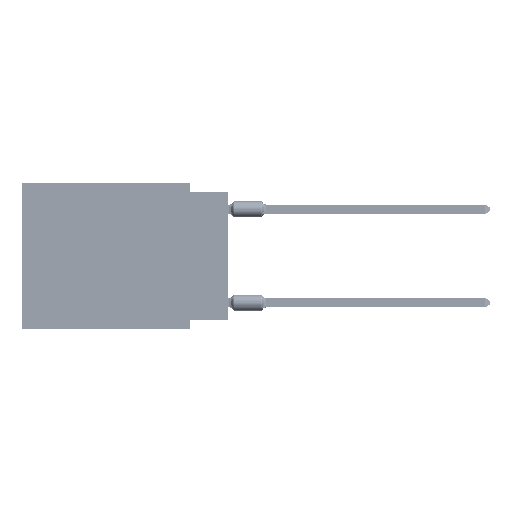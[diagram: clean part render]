
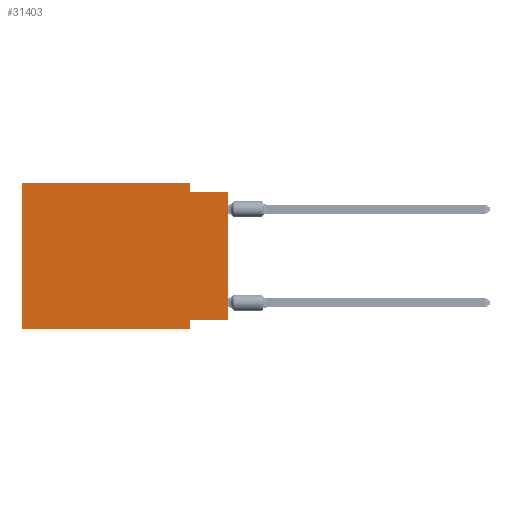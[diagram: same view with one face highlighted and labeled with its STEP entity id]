
A CAD part, left-side view. The second image highlights one B-rep face of the part: STEP entity #31403.
In plain terms, the highlighted planar face has unit normal (-1, 0, 0).
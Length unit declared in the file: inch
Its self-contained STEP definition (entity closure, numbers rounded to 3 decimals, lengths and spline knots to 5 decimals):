
#502 = CARTESIAN_POINT ( 'NONE',  ( 0., 0.1, 0. ) ) ;
#776 = CARTESIAN_POINT ( 'NONE',  ( 0., 0.1, -0.365 ) ) ;
#871 = ORIENTED_EDGE ( 'NONE', *, *, #56005, .F. ) ;
#4397 = DIRECTION ( 'NONE',  ( 0., 0., 1. ) ) ;
#8468 = EDGE_CURVE ( 'NONE', #18296, #77233, #19680, .T. ) ;
#9957 = VERTEX_POINT ( 'NONE', #20885 ) ;
#13483 = DIRECTION ( 'NONE',  ( 0., 0., -1. ) ) ;
#15169 = PLANE ( 'NONE',  #75862 ) ;
#15532 = LINE ( 'NONE', #53945, #24849 ) ;
#15560 = LINE ( 'NONE', #70926, #29838 ) ;
#15585 = DIRECTION ( 'NONE',  ( 0., 0., -1. ) ) ;
#15783 = EDGE_CURVE ( 'NONE', #9957, #73552, #64071, .T. ) ;
#18296 = VERTEX_POINT ( 'NONE', #776 ) ;
#18966 = VERTEX_POINT ( 'NONE', #61311 ) ;
#19308 = CARTESIAN_POINT ( 'NONE',  ( 0., 0.1, -0.39 ) ) ;
#19680 = LINE ( 'NONE', #44871, #29860 ) ;
#19714 = VERTEX_POINT ( 'NONE', #60621 ) ;
#20586 = ORIENTED_EDGE ( 'NONE', *, *, #8468, .F. ) ;
#20684 = CARTESIAN_POINT ( 'NONE',  ( 0., 0.55, 0. ) ) ;
#20786 = DIRECTION ( 'NONE',  ( 0., -1., 0. ) ) ;
#20885 = CARTESIAN_POINT ( 'NONE',  ( 0., 0.55, 0. ) ) ;
#21178 = ORIENTED_EDGE ( 'NONE', *, *, #34280, .T. ) ;
#21198 = CARTESIAN_POINT ( 'NONE',  ( 0., 0.55, -0.39 ) ) ;
#22147 = DIRECTION ( 'NONE',  ( 0., -1., 0. ) ) ;
#22645 = VERTEX_POINT ( 'NONE', #48712 ) ;
#23560 = VECTOR ( 'NONE', #75396, 39.37008 ) ;
#24849 = VECTOR ( 'NONE', #34932, 39.37008 ) ;
#27950 = CARTESIAN_POINT ( 'NONE',  ( 0., 0.55, 0. ) ) ;
#29838 = VECTOR ( 'NONE', #22147, 39.37008 ) ;
#29860 = VECTOR ( 'NONE', #13483, 39.37008 ) ;
#30438 = LINE ( 'NONE', #55647, #67499 ) ;
#30782 = CARTESIAN_POINT ( 'NONE',  ( 0., 0.1, 0. ) ) ;
#31403 = ADVANCED_FACE ( 'NONE', ( #59766 ), #15169, .F. ) ;
#33748 = DIRECTION ( 'NONE',  ( 1., 0., 0. ) ) ;
#34280 = EDGE_CURVE ( 'NONE', #19714, #48058, #78796, .T. ) ;
#34932 = DIRECTION ( 'NONE',  ( 0., 0., 1. ) ) ;
#34978 = CARTESIAN_POINT ( 'NONE',  ( 0., 0., 0. ) ) ;
#36949 = EDGE_CURVE ( 'NONE', #73552, #22645, #68393, .T. ) ;
#37824 = VECTOR ( 'NONE', #4397, 39.37008 ) ;
#40198 = LINE ( 'NONE', #21198, #44003 ) ;
#42339 = ORIENTED_EDGE ( 'NONE', *, *, #52269, .T. ) ;
#44003 = VECTOR ( 'NONE', #20786, 39.37008 ) ;
#44871 = CARTESIAN_POINT ( 'NONE',  ( 0., 0.1, -0.39 ) ) ;
#48058 = VERTEX_POINT ( 'NONE', #59655 ) ;
#48712 = CARTESIAN_POINT ( 'NONE',  ( 0., 0.1, -0.025 ) ) ;
#48901 = VECTOR ( 'NONE', #71110, 39.37008 ) ;
#51818 = EDGE_LOOP ( 'NONE', ( #21178, #871, #59038, #57546, #54740, #42339, #20586, #59491 ) ) ;
#52269 = EDGE_CURVE ( 'NONE', #18966, #77233, #40198, .T. ) ;
#53945 = CARTESIAN_POINT ( 'NONE',  ( 0., 0.55, 0. ) ) ;
#54740 = ORIENTED_EDGE ( 'NONE', *, *, #58139, .F. ) ;
#55647 = CARTESIAN_POINT ( 'NONE',  ( 0., 0., -0.365 ) ) ;
#56005 = EDGE_CURVE ( 'NONE', #22645, #48058, #15560, .T. ) ;
#57546 = ORIENTED_EDGE ( 'NONE', *, *, #15783, .F. ) ;
#58139 = EDGE_CURVE ( 'NONE', #18966, #9957, #15532, .T. ) ;
#59038 = ORIENTED_EDGE ( 'NONE', *, *, #36949, .F. ) ;
#59491 = ORIENTED_EDGE ( 'NONE', *, *, #73820, .F. ) ;
#59655 = CARTESIAN_POINT ( 'NONE',  ( 0., 0., -0.025 ) ) ;
#59766 = FACE_OUTER_BOUND ( 'NONE', #51818, .T. ) ;
#60621 = CARTESIAN_POINT ( 'NONE',  ( 0., 0., -0.365 ) ) ;
#61311 = CARTESIAN_POINT ( 'NONE',  ( 0., 0.55, -0.39 ) ) ;
#64071 = LINE ( 'NONE', #20684, #48901 ) ;
#67499 = VECTOR ( 'NONE', #71488, 39.37008 ) ;
#68393 = LINE ( 'NONE', #30782, #23560 ) ;
#70926 = CARTESIAN_POINT ( 'NONE',  ( 0., 0., -0.025 ) ) ;
#71110 = DIRECTION ( 'NONE',  ( 0., -1., 0. ) ) ;
#71488 = DIRECTION ( 'NONE',  ( 0., 1., 0. ) ) ;
#73552 = VERTEX_POINT ( 'NONE', #502 ) ;
#73820 = EDGE_CURVE ( 'NONE', #19714, #18296, #30438, .T. ) ;
#75396 = DIRECTION ( 'NONE',  ( 0., 0., -1. ) ) ;
#75862 = AXIS2_PLACEMENT_3D ( 'NONE', #27950, #33748, #15585 ) ;
#77233 = VERTEX_POINT ( 'NONE', #19308 ) ;
#78796 = LINE ( 'NONE', #34978, #37824 ) ;
